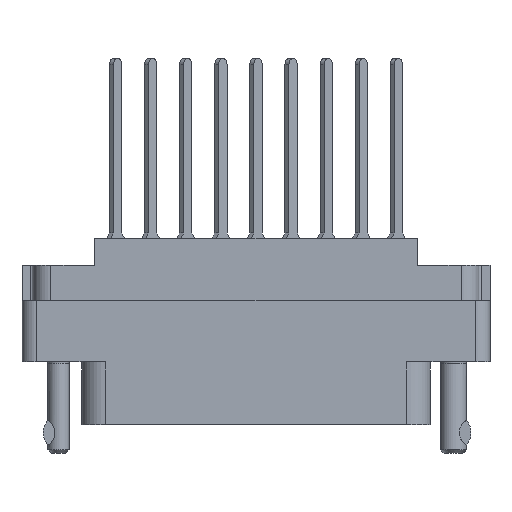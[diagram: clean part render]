
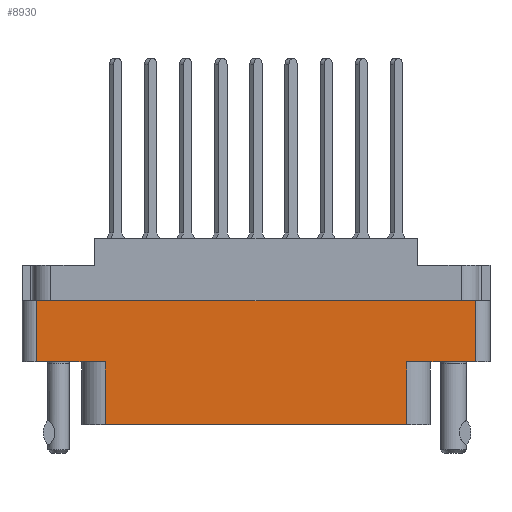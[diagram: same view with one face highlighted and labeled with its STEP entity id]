
A CAD part, front view. The second image highlights one B-rep face of the part: STEP entity #8930.
In plain terms, the highlighted planar face has unit normal (0, -1, 0).
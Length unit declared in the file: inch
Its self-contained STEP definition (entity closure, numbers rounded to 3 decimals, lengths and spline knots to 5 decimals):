
#296 = LINE ( 'NONE', #13944, #40660 ) ;
#2583 = VERTEX_POINT ( 'NONE', #15108 ) ;
#2626 = DIRECTION ( 'NONE',  ( 0., -1., 0. ) ) ;
#3589 = ORIENTED_EDGE ( 'NONE', *, *, #30225, .F. ) ;
#3670 = LINE ( 'NONE', #11406, #40200 ) ;
#5630 = VECTOR ( 'NONE', #28531, 39.37008 ) ;
#6358 = CARTESIAN_POINT ( 'NONE',  ( -0.938, -0.438, -0.529 ) ) ;
#6411 = VERTEX_POINT ( 'NONE', #8860 ) ;
#8860 = CARTESIAN_POINT ( 'NONE',  ( -0.644, -0.438, -0.798 ) ) ;
#8930 = ADVANCED_FACE ( 'NONE', ( #42447 ), #16700, .T. ) ;
#11356 = VERTEX_POINT ( 'NONE', #17654 ) ;
#11406 = CARTESIAN_POINT ( 'NONE',  ( 0.938, -0.438, -0.798 ) ) ;
#11568 = DIRECTION ( 'NONE',  ( 0., 0., -1. ) ) ;
#11570 = EDGE_CURVE ( 'NONE', #35344, #29320, #30651, .T. ) ;
#11715 = VECTOR ( 'NONE', #42562, 39.37008 ) ;
#13944 = CARTESIAN_POINT ( 'NONE',  ( -0.938, -0.438, -0.798 ) ) ;
#15108 = CARTESIAN_POINT ( 'NONE',  ( 0.938, -0.438, -0.268 ) ) ;
#15304 = EDGE_LOOP ( 'NONE', ( #20433, #15954, #33515, #23262, #41835, #17248, #3589, #32512 ) ) ;
#15391 = AXIS2_PLACEMENT_3D ( 'NONE', #23504, #2626, #16240 ) ;
#15679 = DIRECTION ( 'NONE',  ( -1., 0., 0. ) ) ;
#15954 = ORIENTED_EDGE ( 'NONE', *, *, #37892, .T. ) ;
#16037 = EDGE_CURVE ( 'NONE', #24392, #11356, #44719, .T. ) ;
#16240 = DIRECTION ( 'NONE',  ( 0., 0., -1. ) ) ;
#16700 = PLANE ( 'NONE',  #15391 ) ;
#17121 = VERTEX_POINT ( 'NONE', #43728 ) ;
#17248 = ORIENTED_EDGE ( 'NONE', *, *, #37932, .F. ) ;
#17533 = DIRECTION ( 'NONE',  ( 0., 0., 1. ) ) ;
#17575 = LINE ( 'NONE', #18690, #35255 ) ;
#17654 = CARTESIAN_POINT ( 'NONE',  ( -0.644, -0.438, -0.529 ) ) ;
#17834 = VERTEX_POINT ( 'NONE', #35806 ) ;
#18690 = CARTESIAN_POINT ( 'NONE',  ( -0.644, -0.438, -0.529 ) ) ;
#20433 = ORIENTED_EDGE ( 'NONE', *, *, #20449, .T. ) ;
#20449 = EDGE_CURVE ( 'NONE', #11356, #6411, #17575, .T. ) ;
#20555 = EDGE_CURVE ( 'NONE', #17121, #2583, #3670, .T. ) ;
#23262 = ORIENTED_EDGE ( 'NONE', *, *, #29940, .F. ) ;
#23472 = DIRECTION ( 'NONE',  ( 0., 0., 1. ) ) ;
#23504 = CARTESIAN_POINT ( 'NONE',  ( -0.938, -0.438, -0.798 ) ) ;
#24264 = VECTOR ( 'NONE', #38439, 39.37008 ) ;
#24392 = VERTEX_POINT ( 'NONE', #6358 ) ;
#26259 = VECTOR ( 'NONE', #11568, 39.37008 ) ;
#28079 = CARTESIAN_POINT ( 'NONE',  ( -0.938, -0.438, -0.798 ) ) ;
#28407 = CARTESIAN_POINT ( 'NONE',  ( 0., -0.438, -0.529 ) ) ;
#28531 = DIRECTION ( 'NONE',  ( 1., 0., 0. ) ) ;
#29320 = VERTEX_POINT ( 'NONE', #41297 ) ;
#29940 = EDGE_CURVE ( 'NONE', #17121, #35344, #36830, .T. ) ;
#30225 = EDGE_CURVE ( 'NONE', #24392, #17834, #296, .T. ) ;
#30651 = LINE ( 'NONE', #32922, #26259 ) ;
#31293 = VECTOR ( 'NONE', #15679, 39.37008 ) ;
#32512 = ORIENTED_EDGE ( 'NONE', *, *, #16037, .T. ) ;
#32922 = CARTESIAN_POINT ( 'NONE',  ( 0.644, -0.438, -0.529 ) ) ;
#33515 = ORIENTED_EDGE ( 'NONE', *, *, #11570, .F. ) ;
#35255 = VECTOR ( 'NONE', #37257, 39.37008 ) ;
#35344 = VERTEX_POINT ( 'NONE', #43081 ) ;
#35806 = CARTESIAN_POINT ( 'NONE',  ( -0.938, -0.438, -0.268 ) ) ;
#36830 = LINE ( 'NONE', #43940, #31293 ) ;
#37257 = DIRECTION ( 'NONE',  ( 0., 0., -1. ) ) ;
#37892 = EDGE_CURVE ( 'NONE', #6411, #29320, #44854, .T. ) ;
#37932 = EDGE_CURVE ( 'NONE', #17834, #2583, #39327, .T. ) ;
#38439 = DIRECTION ( 'NONE',  ( 1., 0., 0. ) ) ;
#39327 = LINE ( 'NONE', #42400, #11715 ) ;
#40200 = VECTOR ( 'NONE', #23472, 39.37008 ) ;
#40660 = VECTOR ( 'NONE', #17533, 39.37008 ) ;
#41297 = CARTESIAN_POINT ( 'NONE',  ( 0.644, -0.438, -0.798 ) ) ;
#41835 = ORIENTED_EDGE ( 'NONE', *, *, #20555, .T. ) ;
#42400 = CARTESIAN_POINT ( 'NONE',  ( -1., -0.438, -0.268 ) ) ;
#42447 = FACE_OUTER_BOUND ( 'NONE', #15304, .T. ) ;
#42562 = DIRECTION ( 'NONE',  ( 1., 0., 0. ) ) ;
#43081 = CARTESIAN_POINT ( 'NONE',  ( 0.644, -0.438, -0.529 ) ) ;
#43728 = CARTESIAN_POINT ( 'NONE',  ( 0.938, -0.438, -0.529 ) ) ;
#43940 = CARTESIAN_POINT ( 'NONE',  ( 0., -0.438, -0.529 ) ) ;
#44719 = LINE ( 'NONE', #28407, #24264 ) ;
#44854 = LINE ( 'NONE', #28079, #5630 ) ;
